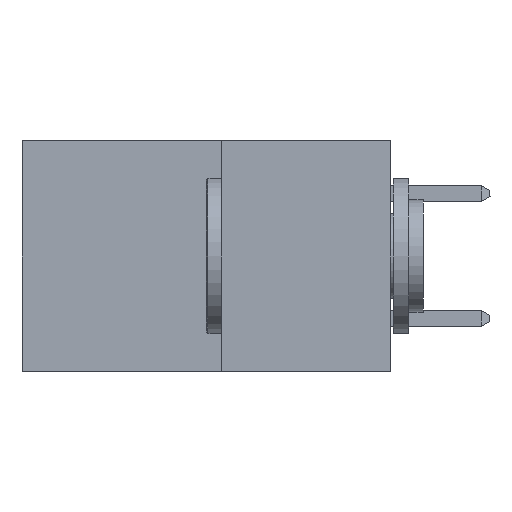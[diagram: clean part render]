
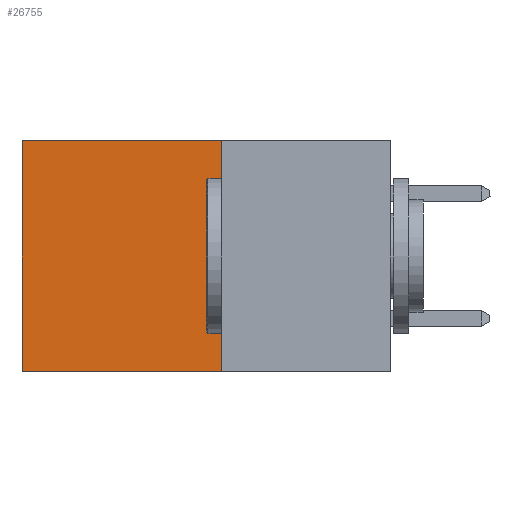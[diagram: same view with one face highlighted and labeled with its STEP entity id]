
A CAD part, left-side view. The second image highlights one B-rep face of the part: STEP entity #26755.
In plain terms, the highlighted planar face has unit normal (-1, 0, 0).
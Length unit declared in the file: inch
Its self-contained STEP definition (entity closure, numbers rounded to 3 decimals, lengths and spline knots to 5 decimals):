
#24 = ORIENTED_EDGE ( 'NONE', *, *, #8680, .F. ) ;
#1155 = ORIENTED_EDGE ( 'NONE', *, *, #2834, .T. ) ;
#1933 = VECTOR ( 'NONE', #27620, 39.37008 ) ;
#2040 = CARTESIAN_POINT ( 'NONE',  ( 0.277, 0.27, 0. ) ) ;
#2834 = EDGE_CURVE ( 'NONE', #29188, #3282, #14398, .T. ) ;
#3282 = VERTEX_POINT ( 'NONE', #25718 ) ;
#3750 = CARTESIAN_POINT ( 'NONE',  ( 0.277, 0.27, -0.37 ) ) ;
#4174 = DIRECTION ( 'NONE',  ( 1., 0., 0. ) ) ;
#4967 = EDGE_CURVE ( 'NONE', #3282, #18206, #5869, .T. ) ;
#5869 = LINE ( 'NONE', #24721, #17540 ) ;
#6838 = CARTESIAN_POINT ( 'NONE',  ( 0.277, 0.27, -0.37 ) ) ;
#7591 = ORIENTED_EDGE ( 'NONE', *, *, #4967, .T. ) ;
#7873 = FACE_OUTER_BOUND ( 'NONE', #16082, .T. ) ;
#8680 = EDGE_CURVE ( 'NONE', #29188, #24224, #23701, .T. ) ;
#12130 = VECTOR ( 'NONE', #20797, 39.37008 ) ;
#14398 = LINE ( 'NONE', #2040, #1933 ) ;
#15194 = CARTESIAN_POINT ( 'NONE',  ( 0.277, 0.27, 0. ) ) ;
#15629 = AXIS2_PLACEMENT_3D ( 'NONE', #18147, #4174, #20464 ) ;
#16082 = EDGE_LOOP ( 'NONE', ( #7591, #25628, #24, #1155 ) ) ;
#16113 = EDGE_CURVE ( 'NONE', #24224, #18206, #25699, .T. ) ;
#17540 = VECTOR ( 'NONE', #24478, 39.37008 ) ;
#18147 = CARTESIAN_POINT ( 'NONE',  ( 0.277, 0.27, -0.37 ) ) ;
#18206 = VERTEX_POINT ( 'NONE', #18416 ) ;
#18416 = CARTESIAN_POINT ( 'NONE',  ( 0.277, 0.59, -0.37 ) ) ;
#19542 = VECTOR ( 'NONE', #27028, 39.37008 ) ;
#20464 = DIRECTION ( 'NONE',  ( 0., 0., -1. ) ) ;
#20797 = DIRECTION ( 'NONE',  ( 0., 0., -1. ) ) ;
#23701 = LINE ( 'NONE', #27772, #12130 ) ;
#24224 = VERTEX_POINT ( 'NONE', #6838 ) ;
#24478 = DIRECTION ( 'NONE',  ( 0., 0., -1. ) ) ;
#24721 = CARTESIAN_POINT ( 'NONE',  ( 0.277, 0.59, -0.37 ) ) ;
#25628 = ORIENTED_EDGE ( 'NONE', *, *, #16113, .F. ) ;
#25699 = LINE ( 'NONE', #3750, #19542 ) ;
#25718 = CARTESIAN_POINT ( 'NONE',  ( 0.277, 0.59, 0. ) ) ;
#26755 = ADVANCED_FACE ( 'NONE', ( #7873 ), #27342, .F. ) ;
#27028 = DIRECTION ( 'NONE',  ( 0., 1., 0. ) ) ;
#27342 = PLANE ( 'NONE',  #15629 ) ;
#27620 = DIRECTION ( 'NONE',  ( 0., 1., 0. ) ) ;
#27772 = CARTESIAN_POINT ( 'NONE',  ( 0.277, 0.27, -0.37 ) ) ;
#29188 = VERTEX_POINT ( 'NONE', #15194 ) ;
